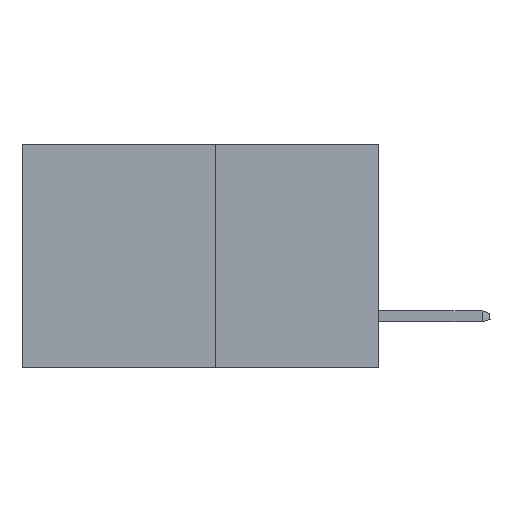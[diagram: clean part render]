
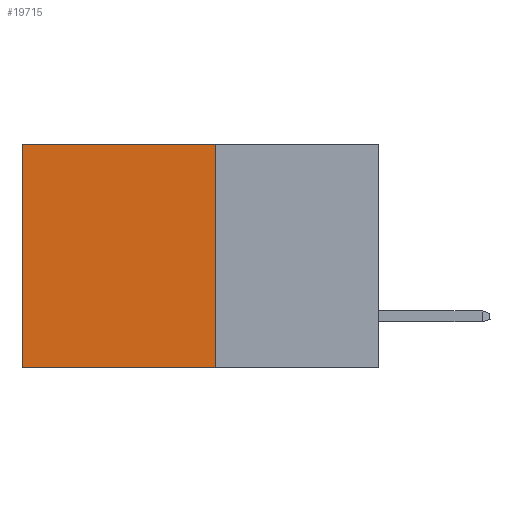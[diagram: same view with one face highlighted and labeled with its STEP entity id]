
A CAD part, left-side view. The second image highlights one B-rep face of the part: STEP entity #19715.
In plain terms, the highlighted planar face has unit normal (-1, 0, 0).
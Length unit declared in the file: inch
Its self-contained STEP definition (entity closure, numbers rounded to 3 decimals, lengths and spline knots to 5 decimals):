
#1293 = VECTOR ( 'NONE', #21383, 39.37008 ) ;
#1407 = CARTESIAN_POINT ( 'NONE',  ( 0.277, 0.59, 0. ) ) ;
#1949 = LINE ( 'NONE', #17276, #1293 ) ;
#3102 = EDGE_LOOP ( 'NONE', ( #21304, #6540, #20061, #12745 ) ) ;
#3641 = CARTESIAN_POINT ( 'NONE',  ( 0.277, 0.27, 0. ) ) ;
#5722 = DIRECTION ( 'NONE',  ( 0., 1., 0. ) ) ;
#6540 = ORIENTED_EDGE ( 'NONE', *, *, #9016, .F. ) ;
#7168 = VERTEX_POINT ( 'NONE', #24134 ) ;
#7575 = EDGE_CURVE ( 'NONE', #17232, #7168, #7868, .T. ) ;
#7868 = LINE ( 'NONE', #18194, #12097 ) ;
#8456 = FACE_OUTER_BOUND ( 'NONE', #3102, .T. ) ;
#9016 = EDGE_CURVE ( 'NONE', #10842, #7168, #20324, .T. ) ;
#9228 = DIRECTION ( 'NONE',  ( 1., 0., 0. ) ) ;
#10842 = VERTEX_POINT ( 'NONE', #13182 ) ;
#11724 = CARTESIAN_POINT ( 'NONE',  ( 0.277, 0.27, -0.37 ) ) ;
#11899 = LINE ( 'NONE', #3641, #12554 ) ;
#12097 = VECTOR ( 'NONE', #18105, 39.37008 ) ;
#12554 = VECTOR ( 'NONE', #5722, 39.37008 ) ;
#12745 = ORIENTED_EDGE ( 'NONE', *, *, #23794, .T. ) ;
#13182 = CARTESIAN_POINT ( 'NONE',  ( 0.277, 0.27, -0.37 ) ) ;
#13794 = DIRECTION ( 'NONE',  ( 0., 1., 0. ) ) ;
#13930 = EDGE_CURVE ( 'NONE', #15370, #10842, #1949, .T. ) ;
#15370 = VERTEX_POINT ( 'NONE', #19919 ) ;
#17232 = VERTEX_POINT ( 'NONE', #1407 ) ;
#17276 = CARTESIAN_POINT ( 'NONE',  ( 0.277, 0.27, -0.37 ) ) ;
#18105 = DIRECTION ( 'NONE',  ( 0., 0., -1. ) ) ;
#18194 = CARTESIAN_POINT ( 'NONE',  ( 0.277, 0.59, -0.37 ) ) ;
#18394 = VECTOR ( 'NONE', #13794, 39.37008 ) ;
#19483 = PLANE ( 'NONE',  #25044 ) ;
#19715 = ADVANCED_FACE ( 'NONE', ( #8456 ), #19483, .F. ) ;
#19919 = CARTESIAN_POINT ( 'NONE',  ( 0.277, 0.27, 0. ) ) ;
#20061 = ORIENTED_EDGE ( 'NONE', *, *, #13930, .F. ) ;
#20324 = LINE ( 'NONE', #11724, #18394 ) ;
#21304 = ORIENTED_EDGE ( 'NONE', *, *, #7575, .T. ) ;
#21383 = DIRECTION ( 'NONE',  ( 0., 0., -1. ) ) ;
#21527 = CARTESIAN_POINT ( 'NONE',  ( 0.277, 0.27, -0.37 ) ) ;
#23569 = DIRECTION ( 'NONE',  ( 0., 0., -1. ) ) ;
#23794 = EDGE_CURVE ( 'NONE', #15370, #17232, #11899, .T. ) ;
#24134 = CARTESIAN_POINT ( 'NONE',  ( 0.277, 0.59, -0.37 ) ) ;
#25044 = AXIS2_PLACEMENT_3D ( 'NONE', #21527, #9228, #23569 ) ;
